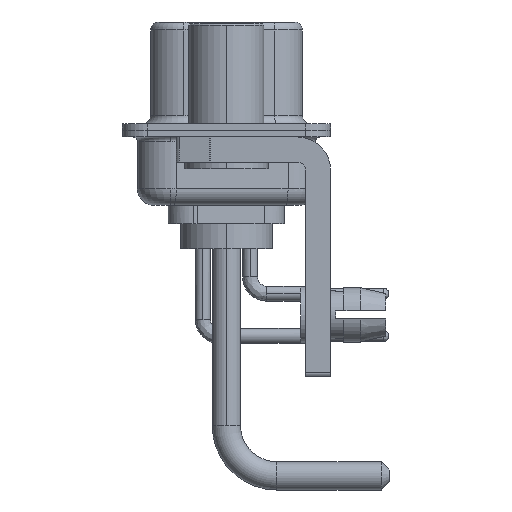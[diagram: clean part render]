
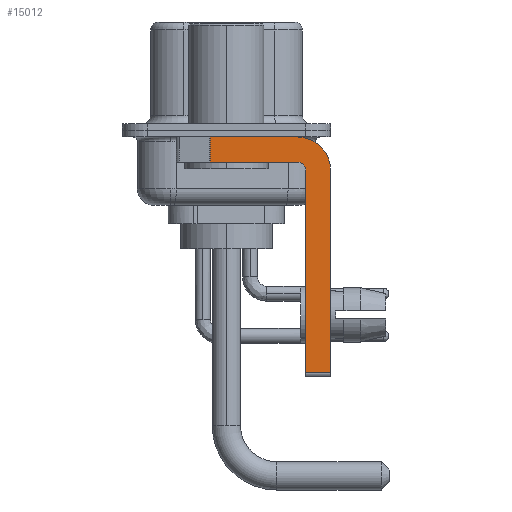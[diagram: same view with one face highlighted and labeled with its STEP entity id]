
A CAD part, left-side view. The second image highlights one B-rep face of the part: STEP entity #15012.
In plain terms, the highlighted planar face has unit normal (-1, 0, 0).
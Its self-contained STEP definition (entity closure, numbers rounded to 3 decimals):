
#275 = CARTESIAN_POINT ( 'NONE',  ( -2.9, -4.75, -2.4 ) ) ;
#400 = LINE ( 'NONE', #17261, #18497 ) ;
#921 = DIRECTION ( 'NONE',  ( 0., -1., 0. ) ) ;
#1099 = EDGE_CURVE ( 'NONE', #23024, #20373, #9480, .T. ) ;
#1178 = VERTEX_POINT ( 'NONE', #275 ) ;
#1497 = LINE ( 'NONE', #15881, #18196 ) ;
#1499 = EDGE_CURVE ( 'NONE', #1178, #8219, #2529, .T. ) ;
#1568 = AXIS2_PLACEMENT_3D ( 'NONE', #3446, #26758, #20168 ) ;
#2529 = CIRCLE ( 'NONE', #4742, 0.5 ) ;
#2705 = LINE ( 'NONE', #25630, #18806 ) ;
#3143 = EDGE_CURVE ( 'NONE', #15493, #15833, #2705, .T. ) ;
#3267 = ORIENTED_EDGE ( 'NONE', *, *, #16945, .F. ) ;
#3430 = ORIENTED_EDGE ( 'NONE', *, *, #1099, .F. ) ;
#3446 = CARTESIAN_POINT ( 'NONE',  ( -2.9, -4.25, -2.4 ) ) ;
#4742 = AXIS2_PLACEMENT_3D ( 'NONE', #15878, #17944, #16136 ) ;
#4791 = EDGE_CURVE ( 'NONE', #8219, #14945, #24847, .T. ) ;
#4947 = DIRECTION ( 'NONE',  ( 0., 0., -1. ) ) ;
#6169 = VECTOR ( 'NONE', #10074, 1000. ) ;
#6353 = CARTESIAN_POINT ( 'NONE',  ( -2.9, -6.25, -2.4 ) ) ;
#6964 = ORIENTED_EDGE ( 'NONE', *, *, #26717, .T. ) ;
#8219 = VERTEX_POINT ( 'NONE', #24297 ) ;
#9480 = CIRCLE ( 'NONE', #1568, 2. ) ;
#10074 = DIRECTION ( 'NONE',  ( 0., 0., -1. ) ) ;
#10142 = VECTOR ( 'NONE', #26044, 1000. ) ;
#12985 = FACE_OUTER_BOUND ( 'NONE', #20668, .T. ) ;
#13365 = CARTESIAN_POINT ( 'NONE',  ( -2.9, -6.25, -2.4 ) ) ;
#14403 = CARTESIAN_POINT ( 'NONE',  ( -2.9, -4.25, -1.9 ) ) ;
#14543 = DIRECTION ( 'NONE',  ( 0., 1., 0. ) ) ;
#14945 = VERTEX_POINT ( 'NONE', #15477 ) ;
#15012 = ADVANCED_FACE ( 'NONE', ( #12985 ), #19271, .F. ) ;
#15285 = CARTESIAN_POINT ( 'NONE',  ( -2.9, -4.25, -2.4 ) ) ;
#15477 = CARTESIAN_POINT ( 'NONE',  ( -2.9, 0.978, -1.9 ) ) ;
#15493 = VERTEX_POINT ( 'NONE', #22371 ) ;
#15833 = VERTEX_POINT ( 'NONE', #17274 ) ;
#15878 = CARTESIAN_POINT ( 'NONE',  ( -2.9, -4.25, -2.4 ) ) ;
#15881 = CARTESIAN_POINT ( 'NONE',  ( -2.9, -4.75, -14.8 ) ) ;
#16136 = DIRECTION ( 'NONE',  ( 0., 0., 1. ) ) ;
#16945 = EDGE_CURVE ( 'NONE', #20373, #15833, #23215, .T. ) ;
#17240 = CARTESIAN_POINT ( 'NONE',  ( -2.9, 0.978, -0.4 ) ) ;
#17261 = CARTESIAN_POINT ( 'NONE',  ( -2.9, 0.978, -1.9 ) ) ;
#17274 = CARTESIAN_POINT ( 'NONE',  ( -2.9, -6.25, -14.55 ) ) ;
#17367 = DIRECTION ( 'NONE',  ( 0., 0., -1. ) ) ;
#17445 = ORIENTED_EDGE ( 'NONE', *, *, #4791, .F. ) ;
#17944 = DIRECTION ( 'NONE',  ( -1., 0., 0. ) ) ;
#18196 = VECTOR ( 'NONE', #24526, 1000. ) ;
#18497 = VECTOR ( 'NONE', #4947, 1000. ) ;
#18806 = VECTOR ( 'NONE', #921, 1000. ) ;
#19271 = PLANE ( 'NONE',  #21402 ) ;
#19562 = DIRECTION ( 'NONE',  ( 1., 0., 0. ) ) ;
#20168 = DIRECTION ( 'NONE',  ( 0., 0., -1. ) ) ;
#20373 = VERTEX_POINT ( 'NONE', #13365 ) ;
#20447 = CARTESIAN_POINT ( 'NONE',  ( -2.9, -4.25, -0.4 ) ) ;
#20668 = EDGE_LOOP ( 'NONE', ( #25453, #6964, #17445, #24082, #22347, #25905, #3267, #3430 ) ) ;
#21402 = AXIS2_PLACEMENT_3D ( 'NONE', #15285, #19562, #17367 ) ;
#21408 = EDGE_CURVE ( 'NONE', #15493, #1178, #1497, .T. ) ;
#21671 = VECTOR ( 'NONE', #14543, 1000. ) ;
#22312 = CARTESIAN_POINT ( 'NONE',  ( -2.9, 3., -0.4 ) ) ;
#22347 = ORIENTED_EDGE ( 'NONE', *, *, #21408, .F. ) ;
#22371 = CARTESIAN_POINT ( 'NONE',  ( -2.9, -4.75, -14.55 ) ) ;
#23024 = VERTEX_POINT ( 'NONE', #20447 ) ;
#23215 = LINE ( 'NONE', #6353, #6169 ) ;
#23812 = VERTEX_POINT ( 'NONE', #17240 ) ;
#23972 = LINE ( 'NONE', #22312, #10142 ) ;
#24082 = ORIENTED_EDGE ( 'NONE', *, *, #1499, .F. ) ;
#24297 = CARTESIAN_POINT ( 'NONE',  ( -2.9, -4.25, -1.9 ) ) ;
#24526 = DIRECTION ( 'NONE',  ( 0., 0., 1. ) ) ;
#24847 = LINE ( 'NONE', #14403, #21671 ) ;
#25102 = EDGE_CURVE ( 'NONE', #23812, #23024, #23972, .T. ) ;
#25453 = ORIENTED_EDGE ( 'NONE', *, *, #25102, .F. ) ;
#25630 = CARTESIAN_POINT ( 'NONE',  ( -2.9, -4.25, -14.55 ) ) ;
#25905 = ORIENTED_EDGE ( 'NONE', *, *, #3143, .T. ) ;
#26044 = DIRECTION ( 'NONE',  ( 0., -1., 0. ) ) ;
#26717 = EDGE_CURVE ( 'NONE', #23812, #14945, #400, .T. ) ;
#26758 = DIRECTION ( 'NONE',  ( 1., 0., 0. ) ) ;
